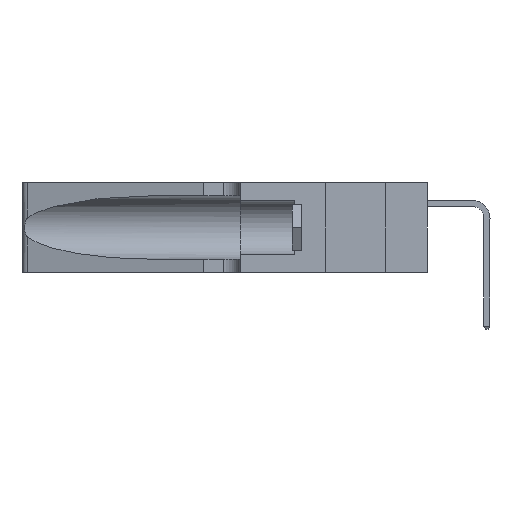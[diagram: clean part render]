
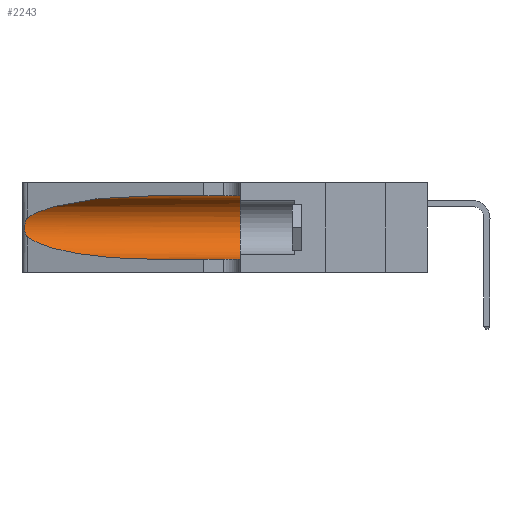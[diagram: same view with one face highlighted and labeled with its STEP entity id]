
A CAD part, left-side view. The second image highlights one B-rep face of the part: STEP entity #2243.
In plain terms, the highlighted cylindrical face has radius 3.308 mm (diameter 6.617 mm), a partial arc.
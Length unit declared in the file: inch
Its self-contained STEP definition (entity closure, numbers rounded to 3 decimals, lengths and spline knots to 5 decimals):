
#341 = VECTOR ( 'NONE', #15176, 39.37008 ) ;
#577 = VERTEX_POINT ( 'NONE', #12790 ) ;
#710 = CARTESIAN_POINT ( 'NONE',  ( 0.18966, 0.96281, 0.31525 ) ) ;
#782 = AXIS2_PLACEMENT_3D ( 'NONE', #4863, #11760, #18377 ) ;
#853 = LINE ( 'NONE', #16743, #341 ) ;
#1113 = CARTESIAN_POINT ( 'NONE',  ( 0.1305, 1.61858, 0.31525 ) ) ;
#1123 = ORIENTED_EDGE ( 'NONE', *, *, #11114, .T. ) ;
#1355 = CARTESIAN_POINT ( 'NONE',  ( 0.26075, 1.23896, 0.178 ) ) ;
#1447 = ORIENTED_EDGE ( 'NONE', *, *, #13656, .T. ) ;
#2243 = ADVANCED_FACE ( 'NONE', ( #3480 ), #2971, .F. ) ;
#2343 = CARTESIAN_POINT ( 'NONE',  ( 0.25487, 1.22718, 0.22369 ) ) ;
#2859 = LINE ( 'NONE', #1113, #10264 ) ;
#2971 = CYLINDRICAL_SURFACE ( 'NONE', #782, 0.13025 ) ;
#2991 = CARTESIAN_POINT ( 'NONE',  ( 0.25856, 1.23593, 0.16098 ) ) ;
#3061 = CIRCLE ( 'NONE', #19653, 0.13025 ) ;
#3480 = FACE_OUTER_BOUND ( 'NONE', #4282, .T. ) ;
#3761 = CARTESIAN_POINT ( 'NONE',  ( 0.1305, 0.72297, 0.05475 ) ) ;
#3802 = DIRECTION ( 'NONE',  ( 0., 1., 0. ) ) ;
#3898 = VERTEX_POINT ( 'NONE', #6219 ) ;
#4282 = EDGE_LOOP ( 'NONE', ( #1447, #17974, #1123, #8538, #18028, #15919 ) ) ;
#4599 = CARTESIAN_POINT ( 'NONE',  ( 0.25639, 1.23186, 0.15144 ) ) ;
#4863 = CARTESIAN_POINT ( 'NONE',  ( 0.1305, 1.61858, 0.185 ) ) ;
#5142 = EDGE_CURVE ( 'NONE', #5893, #8962, #8315, .T. ) ;
#5893 = VERTEX_POINT ( 'NONE', #7641 ) ;
#6164 = CARTESIAN_POINT ( 'NONE',  ( 0.25487, 1.22718, 0.14631 ) ) ;
#6219 = CARTESIAN_POINT ( 'NONE',  ( 0.1305, 0.72297, 0.05475 ) ) ;
#6500 = CARTESIAN_POINT ( 'NONE',  ( 0.1305, 0.72297, 0.31525 ) ) ;
#7641 = CARTESIAN_POINT ( 'NONE',  ( 0.25487, 1.22718, 0.22369 ) ) ;
#8315 = B_SPLINE_CURVE_WITH_KNOTS ( 'NONE', 3,
 ( #10780, #15458, #17041, #18601, #9274, #20148, #10856, #1355, #12434, #2991, #13965, #4599, #15534, #6164 ),
 .UNSPECIFIED., .F., .F.,
 ( 4, 2, 2, 2, 2, 2, 4 ),
 ( 0., 0.00027, 0.00053, 0.00107, 0.0016, 0.00187, 0.00214 ),
 .UNSPECIFIED. ) ;
#8538 = ORIENTED_EDGE ( 'NONE', *, *, #11993, .T. ) ;
#8962 = VERTEX_POINT ( 'NONE', #11076 ) ;
#9274 = CARTESIAN_POINT ( 'NONE',  ( 0.25854, 1.2359, 0.20912 ) ) ;
#10020 = CARTESIAN_POINT ( 'NONE',  ( 0.2373, 1.15595, 0.08982 ) ) ;
#10264 = VECTOR ( 'NONE', #19921, 39.37008 ) ;
#10780 = CARTESIAN_POINT ( 'NONE',  ( 0.25487, 1.22718, 0.22369 ) ) ;
#10856 = CARTESIAN_POINT ( 'NONE',  ( 0.26075, 1.23896, 0.19203 ) ) ;
#11076 = CARTESIAN_POINT ( 'NONE',  ( 0.25487, 1.22718, 0.14631 ) ) ;
#11114 = EDGE_CURVE ( 'NONE', #8962, #3898, #18916, .T. ) ;
#11760 = DIRECTION ( 'NONE',  ( 0., -1., 0. ) ) ;
#11806 = CARTESIAN_POINT ( 'NONE',  ( 0.2373, 1.15595, 0.28018 ) ) ;
#11993 = EDGE_CURVE ( 'NONE', #3898, #15162, #853, .T. ) ;
#12434 = CARTESIAN_POINT ( 'NONE',  ( 0.26017, 1.23833, 0.17102 ) ) ;
#12790 = CARTESIAN_POINT ( 'NONE',  ( 0.1305, 0.35, 0.31525 ) ) ;
#13168 = CARTESIAN_POINT ( 'NONE',  ( 0.18966, 0.96281, 0.05475 ) ) ;
#13203 = CARTESIAN_POINT ( 'NONE',  ( 0.1305, 0.35, 0.185 ) ) ;
#13656 = EDGE_CURVE ( 'NONE', #16045, #5893, #18179, .T. ) ;
#13965 = CARTESIAN_POINT ( 'NONE',  ( 0.25789, 1.23486, 0.15765 ) ) ;
#14608 = EDGE_CURVE ( 'NONE', #16045, #577, #2859, .T. ) ;
#14758 = DIRECTION ( 'NONE',  ( 0., 0., 1. ) ) ;
#15162 = VERTEX_POINT ( 'NONE', #15213 ) ;
#15176 = DIRECTION ( 'NONE',  ( 0., -1., 0. ) ) ;
#15213 = CARTESIAN_POINT ( 'NONE',  ( 0.1305, 0.35, 0.05475 ) ) ;
#15458 = CARTESIAN_POINT ( 'NONE',  ( 0.25555, 1.22994, 0.2215 ) ) ;
#15534 = CARTESIAN_POINT ( 'NONE',  ( 0.25555, 1.22993, 0.14849 ) ) ;
#15919 = ORIENTED_EDGE ( 'NONE', *, *, #14608, .F. ) ;
#16045 = VERTEX_POINT ( 'NONE', #6500 ) ;
#16743 = CARTESIAN_POINT ( 'NONE',  ( 0.1305, 1.61858, 0.05475 ) ) ;
#17041 = CARTESIAN_POINT ( 'NONE',  ( 0.25639, 1.23184, 0.21858 ) ) ;
#17797 = CARTESIAN_POINT ( 'NONE',  ( 0.25487, 1.22718, 0.14631 ) ) ;
#17974 = ORIENTED_EDGE ( 'NONE', *, *, #5142, .T. ) ;
#18028 = ORIENTED_EDGE ( 'NONE', *, *, #19531, .F. ) ;
#18179 =( BOUNDED_CURVE ( )  B_SPLINE_CURVE ( 3, ( #19546, #710, #11806, #2343 ),
 .UNSPECIFIED., .F., .F. ) 
 B_SPLINE_CURVE_WITH_KNOTS ( ( 4, 4 ),
 ( 1.5708, 2.84003 ),
 .UNSPECIFIED. ) 
 CURVE ( )  GEOMETRIC_REPRESENTATION_ITEM ( )  RATIONAL_B_SPLINE_CURVE ( ( 1., 0.87, 0.87, 1. ) ) 
 REPRESENTATION_ITEM ( '' )  );
#18377 = DIRECTION ( 'NONE',  ( 0., 0., -1. ) ) ;
#18601 = CARTESIAN_POINT ( 'NONE',  ( 0.25787, 1.23484, 0.2124 ) ) ;
#18916 =( BOUNDED_CURVE ( )  B_SPLINE_CURVE ( 3, ( #17797, #10020, #13168, #3761 ),
 .UNSPECIFIED., .F., .T. ) 
 B_SPLINE_CURVE_WITH_KNOTS ( ( 4, 4 ),
 ( 3.44316, 4.71239 ),
 .UNSPECIFIED. ) 
 CURVE ( )  GEOMETRIC_REPRESENTATION_ITEM ( )  RATIONAL_B_SPLINE_CURVE ( ( 1., 0.87, 0.87, 1. ) ) 
 REPRESENTATION_ITEM ( '' )  );
#19531 = EDGE_CURVE ( 'NONE', #577, #15162, #3061, .T. ) ;
#19546 = CARTESIAN_POINT ( 'NONE',  ( 0.1305, 0.72297, 0.31525 ) ) ;
#19653 = AXIS2_PLACEMENT_3D ( 'NONE', #13203, #3802, #14758 ) ;
#19921 = DIRECTION ( 'NONE',  ( 0., -1., 0. ) ) ;
#20148 = CARTESIAN_POINT ( 'NONE',  ( 0.26018, 1.23835, 0.19895 ) ) ;
